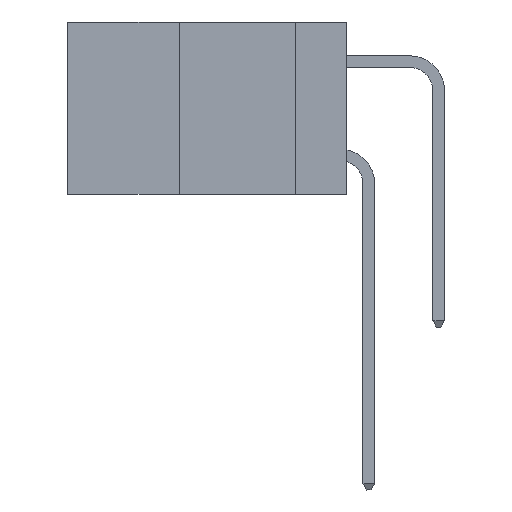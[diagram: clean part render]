
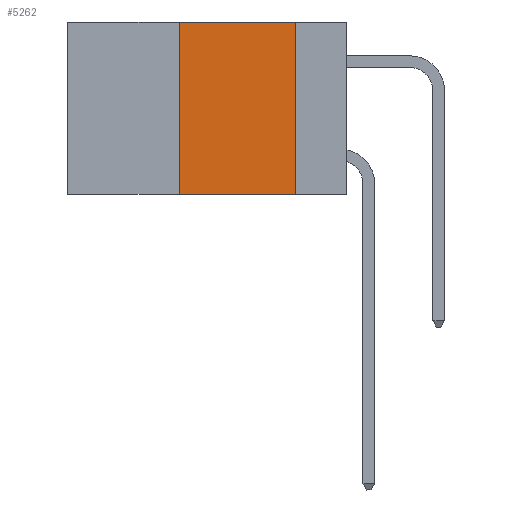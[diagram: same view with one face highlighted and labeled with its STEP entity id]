
A CAD part, left-side view. The second image highlights one B-rep face of the part: STEP entity #5262.
In plain terms, the highlighted planar face has unit normal (-1, 0, 0).
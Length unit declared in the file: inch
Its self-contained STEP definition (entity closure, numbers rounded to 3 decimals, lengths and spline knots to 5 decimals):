
#316 = VECTOR ( 'NONE', #8505, 39.37008 ) ;
#1505 = DIRECTION ( 'NONE',  ( 0., -1., 0. ) ) ;
#1652 = ORIENTED_EDGE ( 'NONE', *, *, #23359, .F. ) ;
#4048 = VERTEX_POINT ( 'NONE', #7248 ) ;
#4322 = LINE ( 'NONE', #6457, #316 ) ;
#5262 = ADVANCED_FACE ( 'NONE', ( #15451 ), #26463, .F. ) ;
#5335 = ORIENTED_EDGE ( 'NONE', *, *, #23684, .F. ) ;
#6245 = AXIS2_PLACEMENT_3D ( 'NONE', #9650, #11677, #7151 ) ;
#6457 = CARTESIAN_POINT ( 'NONE',  ( 0., 0.36, 0. ) ) ;
#6894 = VECTOR ( 'NONE', #13683, 39.37008 ) ;
#7151 = DIRECTION ( 'NONE',  ( 0., 0., -1. ) ) ;
#7248 = CARTESIAN_POINT ( 'NONE',  ( 0., 0.11, 0. ) ) ;
#7374 = EDGE_LOOP ( 'NONE', ( #9373, #5335, #1652, #16182 ) ) ;
#8133 = CARTESIAN_POINT ( 'NONE',  ( 0., 0.36, -0.37 ) ) ;
#8505 = DIRECTION ( 'NONE',  ( 0., 0., 1. ) ) ;
#9268 = LINE ( 'NONE', #22674, #17558 ) ;
#9368 = CARTESIAN_POINT ( 'NONE',  ( 0., 0.6, -0.37 ) ) ;
#9373 = ORIENTED_EDGE ( 'NONE', *, *, #24183, .F. ) ;
#9650 = CARTESIAN_POINT ( 'NONE',  ( 0., 0.6, 0. ) ) ;
#11050 = EDGE_CURVE ( 'NONE', #19319, #26594, #14197, .T. ) ;
#11557 = CARTESIAN_POINT ( 'NONE',  ( 0., 0.11, -0.37 ) ) ;
#11677 = DIRECTION ( 'NONE',  ( 1., 0., 0. ) ) ;
#13589 = DIRECTION ( 'NONE',  ( 0., -1., 0. ) ) ;
#13683 = DIRECTION ( 'NONE',  ( 0., 0., -1. ) ) ;
#14197 = LINE ( 'NONE', #9368, #25202 ) ;
#15451 = FACE_OUTER_BOUND ( 'NONE', #7374, .T. ) ;
#16182 = ORIENTED_EDGE ( 'NONE', *, *, #11050, .T. ) ;
#17066 = CARTESIAN_POINT ( 'NONE',  ( 0., 0.36, 0. ) ) ;
#17558 = VECTOR ( 'NONE', #1505, 39.37008 ) ;
#18058 = CARTESIAN_POINT ( 'NONE',  ( 0., 0.11, 0. ) ) ;
#19319 = VERTEX_POINT ( 'NONE', #8133 ) ;
#21887 = VERTEX_POINT ( 'NONE', #17066 ) ;
#22487 = LINE ( 'NONE', #18058, #6894 ) ;
#22674 = CARTESIAN_POINT ( 'NONE',  ( 0., 0.6, 0. ) ) ;
#23359 = EDGE_CURVE ( 'NONE', #19319, #21887, #4322, .T. ) ;
#23684 = EDGE_CURVE ( 'NONE', #21887, #4048, #9268, .T. ) ;
#24183 = EDGE_CURVE ( 'NONE', #4048, #26594, #22487, .T. ) ;
#25202 = VECTOR ( 'NONE', #13589, 39.37008 ) ;
#26463 = PLANE ( 'NONE',  #6245 ) ;
#26594 = VERTEX_POINT ( 'NONE', #11557 ) ;
